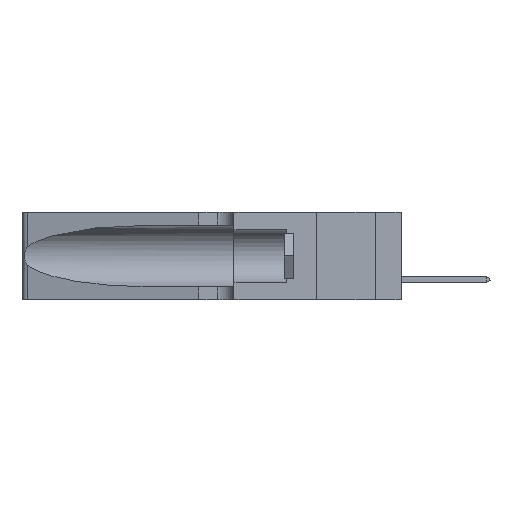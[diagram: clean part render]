
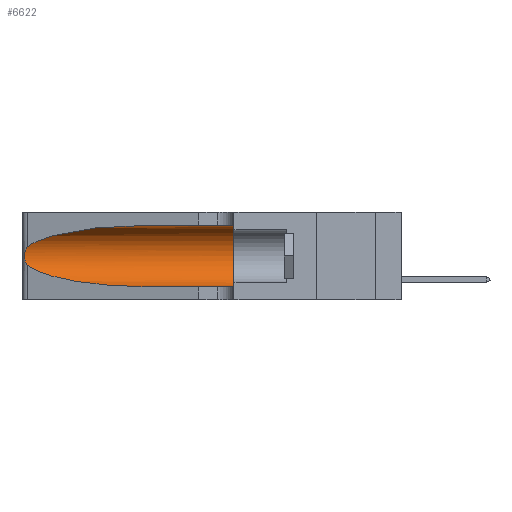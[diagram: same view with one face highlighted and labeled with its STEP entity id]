
A CAD part, left-side view. The second image highlights one B-rep face of the part: STEP entity #6622.
In plain terms, the highlighted cylindrical face has radius 3.308 mm (diameter 6.617 mm), a partial arc.
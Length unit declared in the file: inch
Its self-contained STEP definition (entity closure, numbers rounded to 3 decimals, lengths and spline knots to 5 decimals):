
#477 = CARTESIAN_POINT ( 'NONE',  ( 0.25787, 1.23484, 0.2124 ) ) ;
#593 = CARTESIAN_POINT ( 'NONE',  ( 0.18966, 0.96281, 0.05475 ) ) ;
#1435 = VERTEX_POINT ( 'NONE', #17207 ) ;
#2051 = CARTESIAN_POINT ( 'NONE',  ( 0.1305, 0.35, 0.31525 ) ) ;
#2303 = VERTEX_POINT ( 'NONE', #6147 ) ;
#3716 = B_SPLINE_CURVE_WITH_KNOTS ( 'NONE', 3,
 ( #7092, #7672, #28040, #477, #21158, #35091, #24449, #31041, #41842, #34502, #20868, #7381, #31334, #18020 ),
 .UNSPECIFIED., .F., .F.,
 ( 4, 2, 2, 2, 2, 2, 4 ),
 ( 0., 0.00027, 0.00053, 0.00107, 0.0016, 0.00187, 0.00214 ),
 .UNSPECIFIED. ) ;
#3944 = VERTEX_POINT ( 'NONE', #42781 ) ;
#4057 = CARTESIAN_POINT ( 'NONE',  ( 0.2373, 1.15595, 0.08982 ) ) ;
#4207 = CARTESIAN_POINT ( 'NONE',  ( 0.25487, 1.22718, 0.14631 ) ) ;
#5581 = DIRECTION ( 'NONE',  ( 0., -1., 0. ) ) ;
#6147 = CARTESIAN_POINT ( 'NONE',  ( 0.1305, 0.72297, 0.05475 ) ) ;
#6622 = ADVANCED_FACE ( 'NONE', ( #6628 ), #9305, .F. ) ;
#6628 = FACE_OUTER_BOUND ( 'NONE', #18044, .T. ) ;
#7092 = CARTESIAN_POINT ( 'NONE',  ( 0.25487, 1.22718, 0.22369 ) ) ;
#7381 = CARTESIAN_POINT ( 'NONE',  ( 0.25639, 1.23186, 0.15144 ) ) ;
#7524 = ORIENTED_EDGE ( 'NONE', *, *, #7798, .T. ) ;
#7672 = CARTESIAN_POINT ( 'NONE',  ( 0.25555, 1.22994, 0.2215 ) ) ;
#7798 = EDGE_CURVE ( 'NONE', #3944, #1435, #3716, .T. ) ;
#8759 = LINE ( 'NONE', #33112, #43000 ) ;
#9305 = CYLINDRICAL_SURFACE ( 'NONE', #38607, 0.13025 ) ;
#11072 = CARTESIAN_POINT ( 'NONE',  ( 0.25487, 1.22718, 0.22369 ) ) ;
#13828 =( BOUNDED_CURVE ( )  B_SPLINE_CURVE ( 3, ( #24955, #21678, #28714, #11072 ),
 .UNSPECIFIED., .F., .T. ) 
 B_SPLINE_CURVE_WITH_KNOTS ( ( 4, 4 ),
 ( 1.5708, 2.84003 ),
 .UNSPECIFIED. ) 
 CURVE ( )  GEOMETRIC_REPRESENTATION_ITEM ( )  RATIONAL_B_SPLINE_CURVE ( ( 1., 0.87, 0.87, 1. ) ) 
 REPRESENTATION_ITEM ( '' )  );
#14067 = ORIENTED_EDGE ( 'NONE', *, *, #38656, .T. ) ;
#15123 = EDGE_CURVE ( 'NONE', #1435, #2303, #32252, .T. ) ;
#16730 = CARTESIAN_POINT ( 'NONE',  ( 0.1305, 0.35, 0.05475 ) ) ;
#17207 = CARTESIAN_POINT ( 'NONE',  ( 0.25487, 1.22718, 0.14631 ) ) ;
#17657 = ORIENTED_EDGE ( 'NONE', *, *, #44227, .F. ) ;
#18020 = CARTESIAN_POINT ( 'NONE',  ( 0.25487, 1.22718, 0.14631 ) ) ;
#18044 = EDGE_LOOP ( 'NONE', ( #25610, #7524, #41364, #14067, #17657, #35323 ) ) ;
#19512 = DIRECTION ( 'NONE',  ( 0., -1., 0. ) ) ;
#20868 = CARTESIAN_POINT ( 'NONE',  ( 0.25789, 1.23486, 0.15765 ) ) ;
#21158 = CARTESIAN_POINT ( 'NONE',  ( 0.25854, 1.2359, 0.20912 ) ) ;
#21678 = CARTESIAN_POINT ( 'NONE',  ( 0.18966, 0.96281, 0.31525 ) ) ;
#21966 = EDGE_CURVE ( 'NONE', #43020, #36611, #8759, .T. ) ;
#24449 = CARTESIAN_POINT ( 'NONE',  ( 0.26075, 1.23896, 0.19203 ) ) ;
#24955 = CARTESIAN_POINT ( 'NONE',  ( 0.1305, 0.72297, 0.31525 ) ) ;
#25610 = ORIENTED_EDGE ( 'NONE', *, *, #43910, .T. ) ;
#25824 = CIRCLE ( 'NONE', #36639, 0.13025 ) ;
#26743 = DIRECTION ( 'NONE',  ( 0., -1., 0. ) ) ;
#27866 = CARTESIAN_POINT ( 'NONE',  ( 0.1305, 0.72297, 0.05475 ) ) ;
#28040 = CARTESIAN_POINT ( 'NONE',  ( 0.25639, 1.23184, 0.21858 ) ) ;
#28714 = CARTESIAN_POINT ( 'NONE',  ( 0.2373, 1.15595, 0.28018 ) ) ;
#29558 = VERTEX_POINT ( 'NONE', #16730 ) ;
#29915 = LINE ( 'NONE', #30056, #37950 ) ;
#30056 = CARTESIAN_POINT ( 'NONE',  ( 0.1305, 1.61858, 0.05475 ) ) ;
#30142 = CARTESIAN_POINT ( 'NONE',  ( 0.1305, 0.72297, 0.31525 ) ) ;
#30206 = CARTESIAN_POINT ( 'NONE',  ( 0.1305, 0.35, 0.185 ) ) ;
#31041 = CARTESIAN_POINT ( 'NONE',  ( 0.26075, 1.23896, 0.178 ) ) ;
#31334 = CARTESIAN_POINT ( 'NONE',  ( 0.25555, 1.22993, 0.14849 ) ) ;
#32252 =( BOUNDED_CURVE ( )  B_SPLINE_CURVE ( 3, ( #4207, #4057, #593, #27866 ),
 .UNSPECIFIED., .F., .T. ) 
 B_SPLINE_CURVE_WITH_KNOTS ( ( 4, 4 ),
 ( 3.44316, 4.71239 ),
 .UNSPECIFIED. ) 
 CURVE ( )  GEOMETRIC_REPRESENTATION_ITEM ( )  RATIONAL_B_SPLINE_CURVE ( ( 1., 0.87, 0.87, 1. ) ) 
 REPRESENTATION_ITEM ( '' )  );
#33112 = CARTESIAN_POINT ( 'NONE',  ( 0.1305, 1.61858, 0.31525 ) ) ;
#34502 = CARTESIAN_POINT ( 'NONE',  ( 0.25856, 1.23593, 0.16098 ) ) ;
#35091 = CARTESIAN_POINT ( 'NONE',  ( 0.26018, 1.23835, 0.19895 ) ) ;
#35323 = ORIENTED_EDGE ( 'NONE', *, *, #21966, .F. ) ;
#36494 = DIRECTION ( 'NONE',  ( 0., 1., 0. ) ) ;
#36611 = VERTEX_POINT ( 'NONE', #2051 ) ;
#36639 = AXIS2_PLACEMENT_3D ( 'NONE', #30206, #36494, #43681 ) ;
#37950 = VECTOR ( 'NONE', #26743, 39.37008 ) ;
#38607 = AXIS2_PLACEMENT_3D ( 'NONE', #43488, #5581, #39742 ) ;
#38656 = EDGE_CURVE ( 'NONE', #2303, #29558, #29915, .T. ) ;
#39742 = DIRECTION ( 'NONE',  ( 0., 0., -1. ) ) ;
#41364 = ORIENTED_EDGE ( 'NONE', *, *, #15123, .T. ) ;
#41842 = CARTESIAN_POINT ( 'NONE',  ( 0.26017, 1.23833, 0.17102 ) ) ;
#42781 = CARTESIAN_POINT ( 'NONE',  ( 0.25487, 1.22718, 0.22369 ) ) ;
#43000 = VECTOR ( 'NONE', #19512, 39.37008 ) ;
#43020 = VERTEX_POINT ( 'NONE', #30142 ) ;
#43488 = CARTESIAN_POINT ( 'NONE',  ( 0.1305, 1.61858, 0.185 ) ) ;
#43681 = DIRECTION ( 'NONE',  ( 0., 0., 1. ) ) ;
#43910 = EDGE_CURVE ( 'NONE', #43020, #3944, #13828, .T. ) ;
#44227 = EDGE_CURVE ( 'NONE', #36611, #29558, #25824, .T. ) ;
